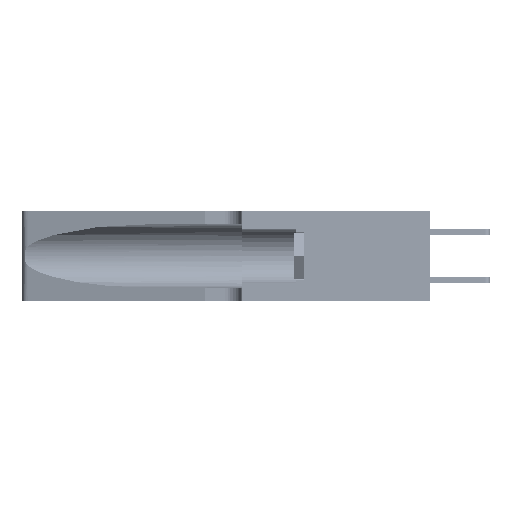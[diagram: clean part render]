
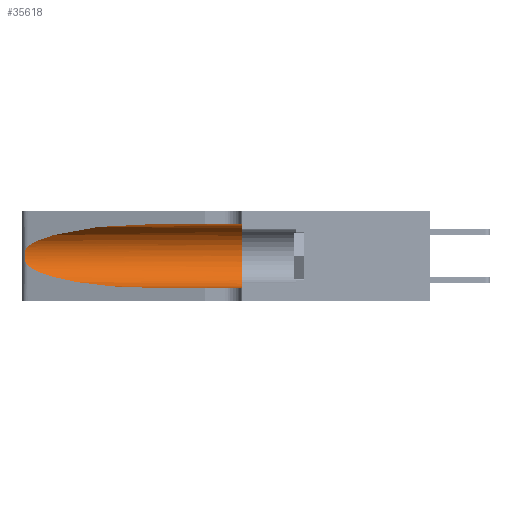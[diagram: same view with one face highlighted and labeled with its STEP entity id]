
A CAD part, left-side view. The second image highlights one B-rep face of the part: STEP entity #35618.
In plain terms, the highlighted cylindrical face has radius 3.308 mm (diameter 6.617 mm), a partial arc.
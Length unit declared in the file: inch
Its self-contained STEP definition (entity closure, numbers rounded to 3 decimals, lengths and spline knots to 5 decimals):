
#492 = VERTEX_POINT ( 'NONE', #39697 ) ;
#536 = B_SPLINE_CURVE_WITH_KNOTS ( 'NONE', 3,
 ( #33032, #26422, #23275, #43589, #6444, #2503, #43445, #6148, #33174, #36570, #29655, #29489, #6301, #9228 ),
 .UNSPECIFIED., .F., .F.,
 ( 4, 2, 2, 2, 2, 2, 4 ),
 ( 0., 0.00027, 0.00053, 0.00107, 0.0016, 0.00187, 0.00214 ),
 .UNSPECIFIED. ) ;
#824 = ORIENTED_EDGE ( 'NONE', *, *, #43544, .F. ) ;
#2503 = CARTESIAN_POINT ( 'NONE',  ( 0.26018, 1.23835, 0.19895 ) ) ;
#5943 = CARTESIAN_POINT ( 'NONE',  ( 0.2373, 1.15595, 0.28018 ) ) ;
#6148 = CARTESIAN_POINT ( 'NONE',  ( 0.26075, 1.23896, 0.178 ) ) ;
#6301 = CARTESIAN_POINT ( 'NONE',  ( 0.25555, 1.22993, 0.14849 ) ) ;
#6348 = ORIENTED_EDGE ( 'NONE', *, *, #24644, .F. ) ;
#6444 = CARTESIAN_POINT ( 'NONE',  ( 0.25854, 1.2359, 0.20912 ) ) ;
#8543 = AXIS2_PLACEMENT_3D ( 'NONE', #21310, #27950, #35159 ) ;
#9201 = CYLINDRICAL_SURFACE ( 'NONE', #28058, 0.13025 ) ;
#9228 = CARTESIAN_POINT ( 'NONE',  ( 0.25487, 1.22718, 0.14631 ) ) ;
#9493 = VERTEX_POINT ( 'NONE', #24022 ) ;
#9767 = FACE_OUTER_BOUND ( 'NONE', #21769, .T. ) ;
#10393 = CARTESIAN_POINT ( 'NONE',  ( 0.1305, 1.61858, 0.185 ) ) ;
#11540 = DIRECTION ( 'NONE',  ( 0., -1., 0. ) ) ;
#12860 = CARTESIAN_POINT ( 'NONE',  ( 0.1305, 0.72297, 0.31525 ) ) ;
#13256 = DIRECTION ( 'NONE',  ( 0., -1., 0. ) ) ;
#13541 = VERTEX_POINT ( 'NONE', #40303 ) ;
#13834 = DIRECTION ( 'NONE',  ( 0., 0., -1. ) ) ;
#15106 = CARTESIAN_POINT ( 'NONE',  ( 0.1305, 0.72297, 0.05475 ) ) ;
#15180 = CARTESIAN_POINT ( 'NONE',  ( 0.1305, 0.72297, 0.05475 ) ) ;
#15204 = CARTESIAN_POINT ( 'NONE',  ( 0.1305, 0.35, 0.31525 ) ) ;
#16453 = VERTEX_POINT ( 'NONE', #34658 ) ;
#17309 = CARTESIAN_POINT ( 'NONE',  ( 0.1305, 1.61858, 0.05475 ) ) ;
#17559 = LINE ( 'NONE', #17309, #37641 ) ;
#18321 = ORIENTED_EDGE ( 'NONE', *, *, #32664, .T. ) ;
#18710 = CARTESIAN_POINT ( 'NONE',  ( 0.18966, 0.96281, 0.05475 ) ) ;
#21310 = CARTESIAN_POINT ( 'NONE',  ( 0.1305, 0.35, 0.185 ) ) ;
#21769 = EDGE_LOOP ( 'NONE', ( #37488, #33313, #18321, #25081, #6348, #824 ) ) ;
#22756 = EDGE_CURVE ( 'NONE', #492, #9493, #24056, .T. ) ;
#23275 = CARTESIAN_POINT ( 'NONE',  ( 0.25639, 1.23184, 0.21858 ) ) ;
#24022 = CARTESIAN_POINT ( 'NONE',  ( 0.25487, 1.22718, 0.22369 ) ) ;
#24056 =( BOUNDED_CURVE ( )  B_SPLINE_CURVE ( 3, ( #12860, #39150, #5943, #29417 ),
 .UNSPECIFIED., .F., .F. ) 
 B_SPLINE_CURVE_WITH_KNOTS ( ( 4, 4 ),
 ( 1.5708, 2.84003 ),
 .UNSPECIFIED. ) 
 CURVE ( )  GEOMETRIC_REPRESENTATION_ITEM ( )  RATIONAL_B_SPLINE_CURVE ( ( 1., 0.87, 0.87, 1. ) ) 
 REPRESENTATION_ITEM ( '' )  );
#24644 = EDGE_CURVE ( 'NONE', #26528, #13541, #42703, .T. ) ;
#25081 = ORIENTED_EDGE ( 'NONE', *, *, #42447, .T. ) ;
#25401 = CARTESIAN_POINT ( 'NONE',  ( 0.25487, 1.22718, 0.14631 ) ) ;
#26083 = VERTEX_POINT ( 'NONE', #15106 ) ;
#26422 = CARTESIAN_POINT ( 'NONE',  ( 0.25555, 1.22994, 0.2215 ) ) ;
#26528 = VERTEX_POINT ( 'NONE', #15204 ) ;
#27578 =( BOUNDED_CURVE ( )  B_SPLINE_CURVE ( 3, ( #25401, #32326, #18710, #15180 ),
 .UNSPECIFIED., .F., .F. ) 
 B_SPLINE_CURVE_WITH_KNOTS ( ( 4, 4 ),
 ( 3.44316, 4.71239 ),
 .UNSPECIFIED. ) 
 CURVE ( )  GEOMETRIC_REPRESENTATION_ITEM ( )  RATIONAL_B_SPLINE_CURVE ( ( 1., 0.87, 0.87, 1. ) ) 
 REPRESENTATION_ITEM ( '' )  );
#27950 = DIRECTION ( 'NONE',  ( 0., 1., 0. ) ) ;
#28058 = AXIS2_PLACEMENT_3D ( 'NONE', #10393, #34068, #13834 ) ;
#28722 = VECTOR ( 'NONE', #13256, 39.37008 ) ;
#29417 = CARTESIAN_POINT ( 'NONE',  ( 0.25487, 1.22718, 0.22369 ) ) ;
#29489 = CARTESIAN_POINT ( 'NONE',  ( 0.25639, 1.23186, 0.15144 ) ) ;
#29655 = CARTESIAN_POINT ( 'NONE',  ( 0.25789, 1.23486, 0.15765 ) ) ;
#32326 = CARTESIAN_POINT ( 'NONE',  ( 0.2373, 1.15595, 0.08982 ) ) ;
#32664 = EDGE_CURVE ( 'NONE', #16453, #26083, #27578, .T. ) ;
#33032 = CARTESIAN_POINT ( 'NONE',  ( 0.25487, 1.22718, 0.22369 ) ) ;
#33174 = CARTESIAN_POINT ( 'NONE',  ( 0.26017, 1.23833, 0.17102 ) ) ;
#33313 = ORIENTED_EDGE ( 'NONE', *, *, #39657, .T. ) ;
#34068 = DIRECTION ( 'NONE',  ( 0., -1., 0. ) ) ;
#34658 = CARTESIAN_POINT ( 'NONE',  ( 0.25487, 1.22718, 0.14631 ) ) ;
#35159 = DIRECTION ( 'NONE',  ( 0., 0., 1. ) ) ;
#35618 = ADVANCED_FACE ( 'NONE', ( #9767 ), #9201, .F. ) ;
#36570 = CARTESIAN_POINT ( 'NONE',  ( 0.25856, 1.23593, 0.16098 ) ) ;
#36627 = LINE ( 'NONE', #43314, #28722 ) ;
#37488 = ORIENTED_EDGE ( 'NONE', *, *, #22756, .T. ) ;
#37641 = VECTOR ( 'NONE', #11540, 39.37008 ) ;
#39150 = CARTESIAN_POINT ( 'NONE',  ( 0.18966, 0.96281, 0.31525 ) ) ;
#39657 = EDGE_CURVE ( 'NONE', #9493, #16453, #536, .T. ) ;
#39697 = CARTESIAN_POINT ( 'NONE',  ( 0.1305, 0.72297, 0.31525 ) ) ;
#40303 = CARTESIAN_POINT ( 'NONE',  ( 0.1305, 0.35, 0.05475 ) ) ;
#42447 = EDGE_CURVE ( 'NONE', #26083, #13541, #17559, .T. ) ;
#42703 = CIRCLE ( 'NONE', #8543, 0.13025 ) ;
#43314 = CARTESIAN_POINT ( 'NONE',  ( 0.1305, 1.61858, 0.31525 ) ) ;
#43445 = CARTESIAN_POINT ( 'NONE',  ( 0.26075, 1.23896, 0.19203 ) ) ;
#43544 = EDGE_CURVE ( 'NONE', #492, #26528, #36627, .T. ) ;
#43589 = CARTESIAN_POINT ( 'NONE',  ( 0.25787, 1.23484, 0.2124 ) ) ;
